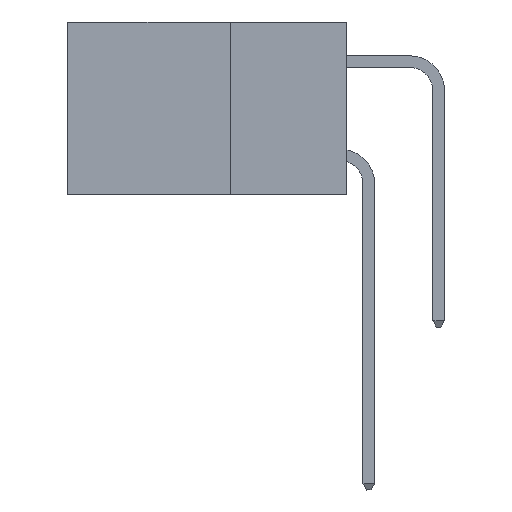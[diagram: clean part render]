
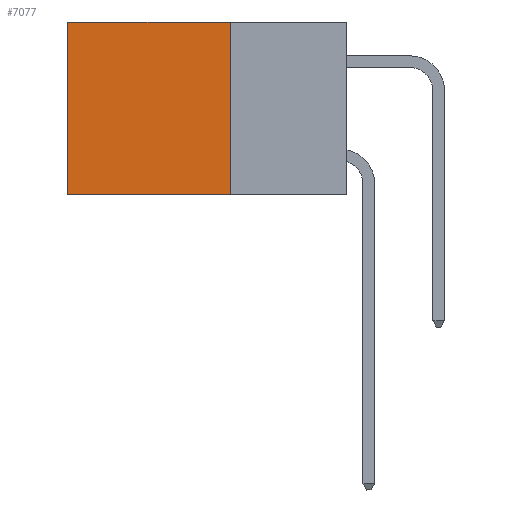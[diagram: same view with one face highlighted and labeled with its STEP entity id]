
A CAD part, left-side view. The second image highlights one B-rep face of the part: STEP entity #7077.
In plain terms, the highlighted planar face has unit normal (-1, 0, 0).
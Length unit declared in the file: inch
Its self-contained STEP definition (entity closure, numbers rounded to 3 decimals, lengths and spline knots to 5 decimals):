
#654 = LINE ( 'NONE', #8103, #3790 ) ;
#1241 = CARTESIAN_POINT ( 'NONE',  ( 0.2875, 0.25, -0.37 ) ) ;
#1799 = ORIENTED_EDGE ( 'NONE', *, *, #6410, .T. ) ;
#2584 = CARTESIAN_POINT ( 'NONE',  ( 0.2875, 0.25, 0. ) ) ;
#2883 = PLANE ( 'NONE',  #11873 ) ;
#3738 = DIRECTION ( 'NONE',  ( 0., 0., -1. ) ) ;
#3790 = VECTOR ( 'NONE', #14988, 39.37008 ) ;
#3955 = FACE_OUTER_BOUND ( 'NONE', #11182, .T. ) ;
#4029 = CARTESIAN_POINT ( 'NONE',  ( 0.2875, 0.25, 0. ) ) ;
#4753 = VERTEX_POINT ( 'NONE', #9663 ) ;
#5179 = DIRECTION ( 'NONE',  ( 1., 0., 0. ) ) ;
#5234 = EDGE_CURVE ( 'NONE', #5674, #4753, #7080, .T. ) ;
#5638 = CARTESIAN_POINT ( 'NONE',  ( 0.2875, 0.6, 0. ) ) ;
#5674 = VERTEX_POINT ( 'NONE', #5638 ) ;
#6060 = CARTESIAN_POINT ( 'NONE',  ( 0.2875, 0.6, 0. ) ) ;
#6192 = CARTESIAN_POINT ( 'NONE',  ( 0.2875, 0.25, 0. ) ) ;
#6383 = EDGE_CURVE ( 'NONE', #6471, #4753, #13331, .T. ) ;
#6410 = EDGE_CURVE ( 'NONE', #11842, #5674, #654, .T. ) ;
#6471 = VERTEX_POINT ( 'NONE', #1241 ) ;
#6870 = VECTOR ( 'NONE', #9217, 39.37008 ) ;
#6934 = CARTESIAN_POINT ( 'NONE',  ( 0.2875, 0.25, -0.37 ) ) ;
#7077 = ADVANCED_FACE ( 'NONE', ( #3955 ), #2883, .F. ) ;
#7080 = LINE ( 'NONE', #6060, #12826 ) ;
#8103 = CARTESIAN_POINT ( 'NONE',  ( 0.2875, 0.25, 0. ) ) ;
#8237 = ORIENTED_EDGE ( 'NONE', *, *, #6383, .F. ) ;
#9217 = DIRECTION ( 'NONE',  ( 0., 1., 0. ) ) ;
#9563 = DIRECTION ( 'NONE',  ( 0., 0., -1. ) ) ;
#9663 = CARTESIAN_POINT ( 'NONE',  ( 0.2875, 0.6, -0.37 ) ) ;
#10911 = ORIENTED_EDGE ( 'NONE', *, *, #12420, .F. ) ;
#11182 = EDGE_LOOP ( 'NONE', ( #12913, #8237, #10911, #1799 ) ) ;
#11842 = VERTEX_POINT ( 'NONE', #6192 ) ;
#11873 = AXIS2_PLACEMENT_3D ( 'NONE', #4029, #5179, #13228 ) ;
#12420 = EDGE_CURVE ( 'NONE', #11842, #6471, #13582, .T. ) ;
#12826 = VECTOR ( 'NONE', #9563, 39.37008 ) ;
#12913 = ORIENTED_EDGE ( 'NONE', *, *, #5234, .T. ) ;
#13225 = VECTOR ( 'NONE', #3738, 39.37008 ) ;
#13228 = DIRECTION ( 'NONE',  ( 0., 0., -1. ) ) ;
#13331 = LINE ( 'NONE', #6934, #6870 ) ;
#13582 = LINE ( 'NONE', #2584, #13225 ) ;
#14988 = DIRECTION ( 'NONE',  ( 0., 1., 0. ) ) ;
